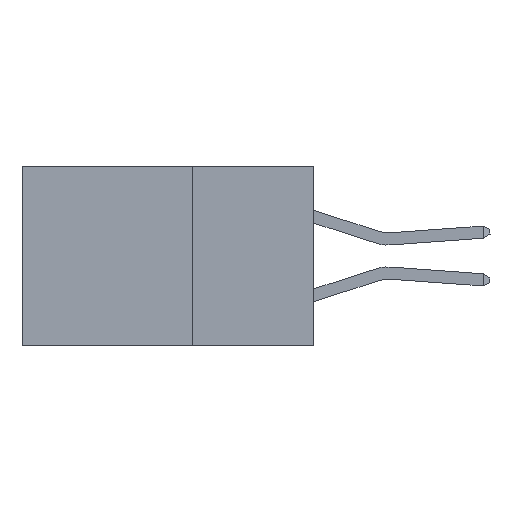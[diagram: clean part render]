
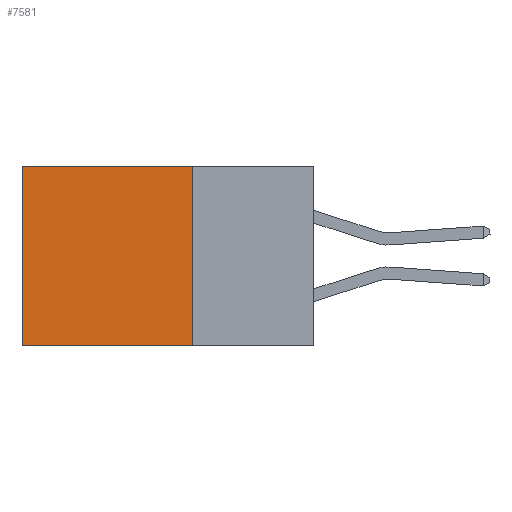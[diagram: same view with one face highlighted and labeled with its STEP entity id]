
A CAD part, left-side view. The second image highlights one B-rep face of the part: STEP entity #7581.
In plain terms, the highlighted planar face has unit normal (-1, 0, 0).
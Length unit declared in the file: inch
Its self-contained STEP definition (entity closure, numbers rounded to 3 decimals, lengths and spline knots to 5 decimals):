
#59 = VECTOR ( 'NONE', #141, 39.37008 ) ;
#141 = DIRECTION ( 'NONE',  ( 0., 0., -1. ) ) ;
#382 = LINE ( 'NONE', #1157, #2003 ) ;
#1157 = CARTESIAN_POINT ( 'NONE',  ( 0.2875, 0.25, -0.37 ) ) ;
#1231 = VERTEX_POINT ( 'NONE', #5520 ) ;
#1579 = VERTEX_POINT ( 'NONE', #11510 ) ;
#1683 = ORIENTED_EDGE ( 'NONE', *, *, #5098, .F. ) ;
#2003 = VECTOR ( 'NONE', #2334, 39.37008 ) ;
#2334 = DIRECTION ( 'NONE',  ( 0., 1., 0. ) ) ;
#2531 = DIRECTION ( 'NONE',  ( 1., 0., 0. ) ) ;
#3956 = ORIENTED_EDGE ( 'NONE', *, *, #6172, .F. ) ;
#4053 = EDGE_CURVE ( 'NONE', #1231, #12046, #7558, .T. ) ;
#4444 = VECTOR ( 'NONE', #16185, 39.37008 ) ;
#4648 = LINE ( 'NONE', #13659, #4444 ) ;
#5098 = EDGE_CURVE ( 'NONE', #1579, #16210, #4648, .T. ) ;
#5446 = ORIENTED_EDGE ( 'NONE', *, *, #4053, .T. ) ;
#5520 = CARTESIAN_POINT ( 'NONE',  ( 0.2875, 0.6, 0. ) ) ;
#6172 = EDGE_CURVE ( 'NONE', #16210, #12046, #382, .T. ) ;
#6502 = CARTESIAN_POINT ( 'NONE',  ( 0.2875, 0.25, -0.37 ) ) ;
#6921 = DIRECTION ( 'NONE',  ( 0., 1., 0. ) ) ;
#7558 = LINE ( 'NONE', #7950, #59 ) ;
#7581 = ADVANCED_FACE ( 'NONE', ( #10327 ), #11094, .F. ) ;
#7950 = CARTESIAN_POINT ( 'NONE',  ( 0.2875, 0.6, 0. ) ) ;
#8079 = CARTESIAN_POINT ( 'NONE',  ( 0.2875, 0.25, 0. ) ) ;
#9055 = DIRECTION ( 'NONE',  ( 0., 0., -1. ) ) ;
#9952 = CARTESIAN_POINT ( 'NONE',  ( 0.2875, 0.6, -0.37 ) ) ;
#10327 = FACE_OUTER_BOUND ( 'NONE', #11486, .T. ) ;
#10388 = LINE ( 'NONE', #8079, #11810 ) ;
#11094 = PLANE ( 'NONE',  #11588 ) ;
#11486 = EDGE_LOOP ( 'NONE', ( #5446, #3956, #1683, #14136 ) ) ;
#11510 = CARTESIAN_POINT ( 'NONE',  ( 0.2875, 0.25, 0. ) ) ;
#11588 = AXIS2_PLACEMENT_3D ( 'NONE', #13732, #2531, #9055 ) ;
#11791 = EDGE_CURVE ( 'NONE', #1579, #1231, #10388, .T. ) ;
#11810 = VECTOR ( 'NONE', #6921, 39.37008 ) ;
#12046 = VERTEX_POINT ( 'NONE', #9952 ) ;
#13659 = CARTESIAN_POINT ( 'NONE',  ( 0.2875, 0.25, 0. ) ) ;
#13732 = CARTESIAN_POINT ( 'NONE',  ( 0.2875, 0.25, 0. ) ) ;
#14136 = ORIENTED_EDGE ( 'NONE', *, *, #11791, .T. ) ;
#16185 = DIRECTION ( 'NONE',  ( 0., 0., -1. ) ) ;
#16210 = VERTEX_POINT ( 'NONE', #6502 ) ;
